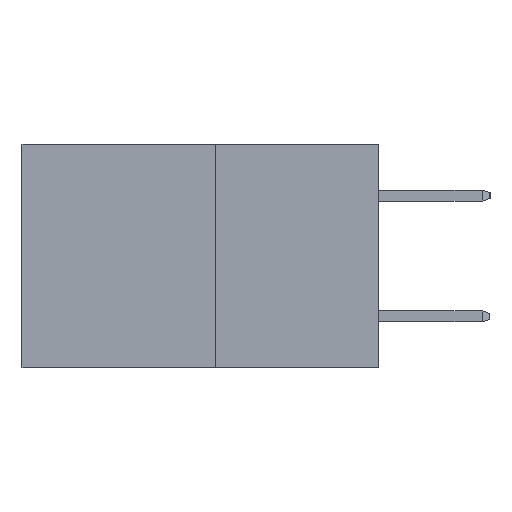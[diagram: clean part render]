
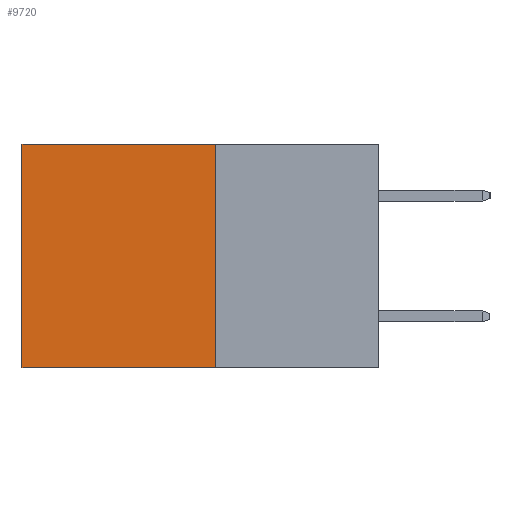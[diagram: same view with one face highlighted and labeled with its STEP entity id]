
A CAD part, left-side view. The second image highlights one B-rep face of the part: STEP entity #9720.
In plain terms, the highlighted planar face has unit normal (-1, 0, 0).
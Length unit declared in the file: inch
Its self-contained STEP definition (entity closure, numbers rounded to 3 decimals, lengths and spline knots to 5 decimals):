
#188 = CARTESIAN_POINT ( 'NONE',  ( 0.277, 0.59, 0. ) ) ;
#482 = VERTEX_POINT ( 'NONE', #1163 ) ;
#716 = CARTESIAN_POINT ( 'NONE',  ( 0.277, 0.27, -0.37 ) ) ;
#1163 = CARTESIAN_POINT ( 'NONE',  ( 0.277, 0.27, -0.37 ) ) ;
#1505 = CARTESIAN_POINT ( 'NONE',  ( 0.277, 0.59, -0.37 ) ) ;
#2268 = DIRECTION ( 'NONE',  ( 0., 1., 0. ) ) ;
#2336 = EDGE_CURVE ( 'NONE', #8974, #482, #2669, .T. ) ;
#2422 = VERTEX_POINT ( 'NONE', #5660 ) ;
#2594 = VECTOR ( 'NONE', #2268, 39.37008 ) ;
#2669 = LINE ( 'NONE', #6598, #7523 ) ;
#3289 = VECTOR ( 'NONE', #10913, 39.37008 ) ;
#3405 = DIRECTION ( 'NONE',  ( 0., 0., -1. ) ) ;
#3573 = LINE ( 'NONE', #1505, #3289 ) ;
#4361 = ORIENTED_EDGE ( 'NONE', *, *, #9939, .F. ) ;
#4649 = ORIENTED_EDGE ( 'NONE', *, *, #10815, .T. ) ;
#4723 = LINE ( 'NONE', #6285, #11169 ) ;
#5085 = CARTESIAN_POINT ( 'NONE',  ( 0.277, 0.27, 0. ) ) ;
#5431 = VERTEX_POINT ( 'NONE', #188 ) ;
#5660 = CARTESIAN_POINT ( 'NONE',  ( 0.277, 0.59, -0.37 ) ) ;
#6121 = DIRECTION ( 'NONE',  ( 0., 0., -1. ) ) ;
#6247 = DIRECTION ( 'NONE',  ( 0., 1., 0. ) ) ;
#6285 = CARTESIAN_POINT ( 'NONE',  ( 0.277, 0.27, -0.37 ) ) ;
#6598 = CARTESIAN_POINT ( 'NONE',  ( 0.277, 0.27, -0.37 ) ) ;
#6747 = AXIS2_PLACEMENT_3D ( 'NONE', #716, #8498, #3405 ) ;
#7075 = EDGE_LOOP ( 'NONE', ( #8568, #4361, #11088, #4649 ) ) ;
#7352 = FACE_OUTER_BOUND ( 'NONE', #7075, .T. ) ;
#7523 = VECTOR ( 'NONE', #6121, 39.37008 ) ;
#8454 = PLANE ( 'NONE',  #6747 ) ;
#8498 = DIRECTION ( 'NONE',  ( 1., 0., 0. ) ) ;
#8568 = ORIENTED_EDGE ( 'NONE', *, *, #10903, .T. ) ;
#8615 = LINE ( 'NONE', #9137, #2594 ) ;
#8974 = VERTEX_POINT ( 'NONE', #5085 ) ;
#9137 = CARTESIAN_POINT ( 'NONE',  ( 0.277, 0.27, 0. ) ) ;
#9720 = ADVANCED_FACE ( 'NONE', ( #7352 ), #8454, .F. ) ;
#9939 = EDGE_CURVE ( 'NONE', #482, #2422, #4723, .T. ) ;
#10815 = EDGE_CURVE ( 'NONE', #8974, #5431, #8615, .T. ) ;
#10903 = EDGE_CURVE ( 'NONE', #5431, #2422, #3573, .T. ) ;
#10913 = DIRECTION ( 'NONE',  ( 0., 0., -1. ) ) ;
#11088 = ORIENTED_EDGE ( 'NONE', *, *, #2336, .F. ) ;
#11169 = VECTOR ( 'NONE', #6247, 39.37008 ) ;
